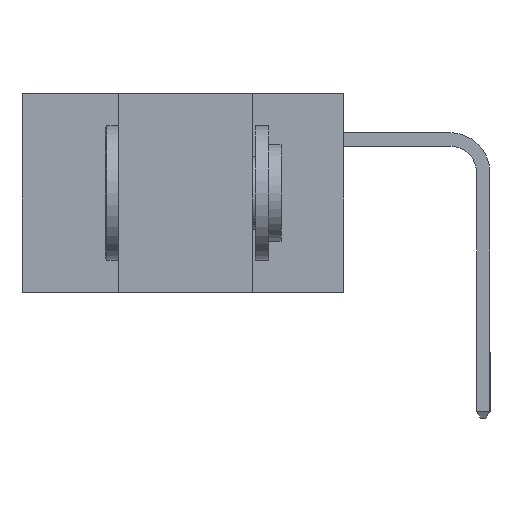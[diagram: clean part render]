
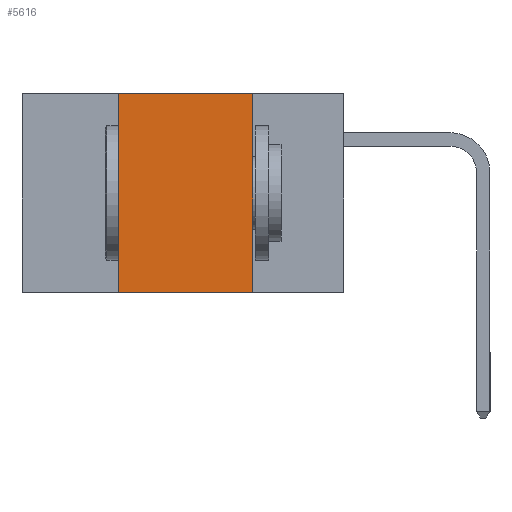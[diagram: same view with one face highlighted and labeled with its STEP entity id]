
A CAD part, left-side view. The second image highlights one B-rep face of the part: STEP entity #5616.
In plain terms, the highlighted planar face has unit normal (-1, 0, 0).
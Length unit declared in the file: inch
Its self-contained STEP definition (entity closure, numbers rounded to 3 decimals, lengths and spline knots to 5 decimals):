
#516 = EDGE_CURVE ( 'NONE', #16972, #19380, #2015, .T. ) ;
#2015 = LINE ( 'NONE', #10624, #15314 ) ;
#2181 = DIRECTION ( 'NONE',  ( 0., -1., 0. ) ) ;
#2410 = EDGE_CURVE ( 'NONE', #6858, #6703, #11498, .T. ) ;
#2743 = LINE ( 'NONE', #9030, #20538 ) ;
#2896 = ORIENTED_EDGE ( 'NONE', *, *, #2410, .F. ) ;
#5616 = ADVANCED_FACE ( 'NONE', ( #21212 ), #6103, .F. ) ;
#6103 = PLANE ( 'NONE',  #11197 ) ;
#6703 = VERTEX_POINT ( 'NONE', #8035 ) ;
#6709 = ORIENTED_EDGE ( 'NONE', *, *, #11489, .F. ) ;
#6829 = VECTOR ( 'NONE', #11136, 39.37008 ) ;
#6858 = VERTEX_POINT ( 'NONE', #15669 ) ;
#6947 = EDGE_CURVE ( 'NONE', #6858, #19380, #10216, .T. ) ;
#8008 = ORIENTED_EDGE ( 'NONE', *, *, #6947, .T. ) ;
#8035 = CARTESIAN_POINT ( 'NONE',  ( 0., 0.42, 0. ) ) ;
#8323 = DIRECTION ( 'NONE',  ( 0., 0., -1. ) ) ;
#9030 = CARTESIAN_POINT ( 'NONE',  ( 0., 0.6, 0. ) ) ;
#9412 = CARTESIAN_POINT ( 'NONE',  ( 0., 0.17, 0. ) ) ;
#9898 = ORIENTED_EDGE ( 'NONE', *, *, #516, .F. ) ;
#10216 = LINE ( 'NONE', #20237, #12379 ) ;
#10624 = CARTESIAN_POINT ( 'NONE',  ( 0., 0.17, 0. ) ) ;
#11090 = CARTESIAN_POINT ( 'NONE',  ( 0., 0.42, 0. ) ) ;
#11132 = DIRECTION ( 'NONE',  ( 0., 0., -1. ) ) ;
#11136 = DIRECTION ( 'NONE',  ( 0., 0., 1. ) ) ;
#11138 = DIRECTION ( 'NONE',  ( 1., 0., 0. ) ) ;
#11197 = AXIS2_PLACEMENT_3D ( 'NONE', #21487, #11138, #11132 ) ;
#11489 = EDGE_CURVE ( 'NONE', #6703, #16972, #2743, .T. ) ;
#11498 = LINE ( 'NONE', #11090, #6829 ) ;
#12379 = VECTOR ( 'NONE', #20155, 39.37008 ) ;
#12607 = CARTESIAN_POINT ( 'NONE',  ( 0., 0.17, -0.37 ) ) ;
#15314 = VECTOR ( 'NONE', #8323, 39.37008 ) ;
#15669 = CARTESIAN_POINT ( 'NONE',  ( 0., 0.42, -0.37 ) ) ;
#16972 = VERTEX_POINT ( 'NONE', #9412 ) ;
#17255 = EDGE_LOOP ( 'NONE', ( #9898, #6709, #2896, #8008 ) ) ;
#19380 = VERTEX_POINT ( 'NONE', #12607 ) ;
#20155 = DIRECTION ( 'NONE',  ( 0., -1., 0. ) ) ;
#20237 = CARTESIAN_POINT ( 'NONE',  ( 0., 0.6, -0.37 ) ) ;
#20538 = VECTOR ( 'NONE', #2181, 39.37008 ) ;
#21212 = FACE_OUTER_BOUND ( 'NONE', #17255, .T. ) ;
#21487 = CARTESIAN_POINT ( 'NONE',  ( 0., 0.6, 0. ) ) ;
